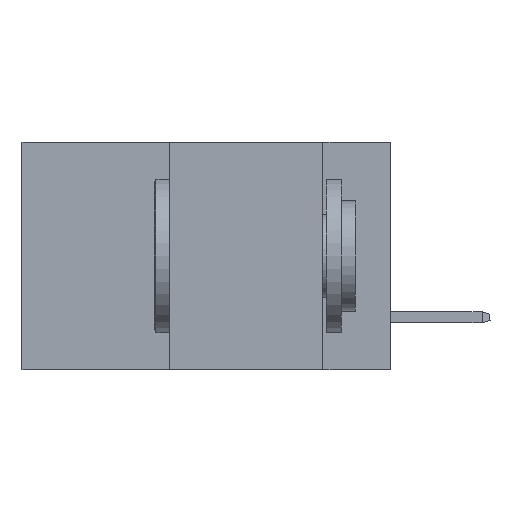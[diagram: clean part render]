
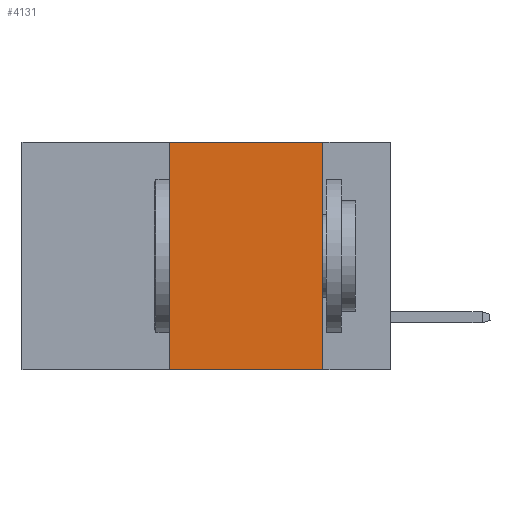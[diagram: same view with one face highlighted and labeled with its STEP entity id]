
A CAD part, left-side view. The second image highlights one B-rep face of the part: STEP entity #4131.
In plain terms, the highlighted planar face has unit normal (-1, 0, 0).
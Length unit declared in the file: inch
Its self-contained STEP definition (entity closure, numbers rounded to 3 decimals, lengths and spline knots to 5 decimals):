
#282 = ORIENTED_EDGE ( 'NONE', *, *, #621, .T. ) ;
#345 = LINE ( 'NONE', #6904, #9862 ) ;
#481 = FACE_OUTER_BOUND ( 'NONE', #8357, .T. ) ;
#621 = EDGE_CURVE ( 'NONE', #7251, #10926, #5100, .T. ) ;
#701 = DIRECTION ( 'NONE',  ( 0., -1., 0. ) ) ;
#1144 = CARTESIAN_POINT ( 'NONE',  ( 0., 0.36, 0. ) ) ;
#1253 = CARTESIAN_POINT ( 'NONE',  ( 0., 0.6, 0. ) ) ;
#1333 = CARTESIAN_POINT ( 'NONE',  ( 0., 0.6, -0.37 ) ) ;
#2165 = AXIS2_PLACEMENT_3D ( 'NONE', #1253, #5952, #10498 ) ;
#3409 = EDGE_CURVE ( 'NONE', #7251, #10370, #345, .T. ) ;
#3722 = ORIENTED_EDGE ( 'NONE', *, *, #3409, .F. ) ;
#4131 = ADVANCED_FACE ( 'NONE', ( #481 ), #4834, .F. ) ;
#4416 = DIRECTION ( 'NONE',  ( 0., -1., 0. ) ) ;
#4834 = PLANE ( 'NONE',  #2165 ) ;
#4962 = VERTEX_POINT ( 'NONE', #8634 ) ;
#5100 = LINE ( 'NONE', #1333, #5959 ) ;
#5307 = CARTESIAN_POINT ( 'NONE',  ( 0., 0.6, 0. ) ) ;
#5467 = EDGE_CURVE ( 'NONE', #4962, #10926, #7201, .T. ) ;
#5878 = DIRECTION ( 'NONE',  ( 0., 0., 1. ) ) ;
#5952 = DIRECTION ( 'NONE',  ( 1., 0., 0. ) ) ;
#5959 = VECTOR ( 'NONE', #701, 39.37008 ) ;
#6904 = CARTESIAN_POINT ( 'NONE',  ( 0., 0.36, 0. ) ) ;
#7201 = LINE ( 'NONE', #11234, #11851 ) ;
#7251 = VERTEX_POINT ( 'NONE', #10398 ) ;
#7707 = VECTOR ( 'NONE', #4416, 39.37008 ) ;
#8357 = EDGE_LOOP ( 'NONE', ( #11959, #10846, #3722, #282 ) ) ;
#8634 = CARTESIAN_POINT ( 'NONE',  ( 0., 0.11, 0. ) ) ;
#8876 = CARTESIAN_POINT ( 'NONE',  ( 0., 0.11, -0.37 ) ) ;
#9449 = DIRECTION ( 'NONE',  ( 0., 0., -1. ) ) ;
#9862 = VECTOR ( 'NONE', #5878, 39.37008 ) ;
#10370 = VERTEX_POINT ( 'NONE', #1144 ) ;
#10398 = CARTESIAN_POINT ( 'NONE',  ( 0., 0.36, -0.37 ) ) ;
#10498 = DIRECTION ( 'NONE',  ( 0., 0., -1. ) ) ;
#10846 = ORIENTED_EDGE ( 'NONE', *, *, #11661, .F. ) ;
#10926 = VERTEX_POINT ( 'NONE', #8876 ) ;
#11234 = CARTESIAN_POINT ( 'NONE',  ( 0., 0.11, 0. ) ) ;
#11661 = EDGE_CURVE ( 'NONE', #10370, #4962, #11770, .T. ) ;
#11770 = LINE ( 'NONE', #5307, #7707 ) ;
#11851 = VECTOR ( 'NONE', #9449, 39.37008 ) ;
#11959 = ORIENTED_EDGE ( 'NONE', *, *, #5467, .F. ) ;
